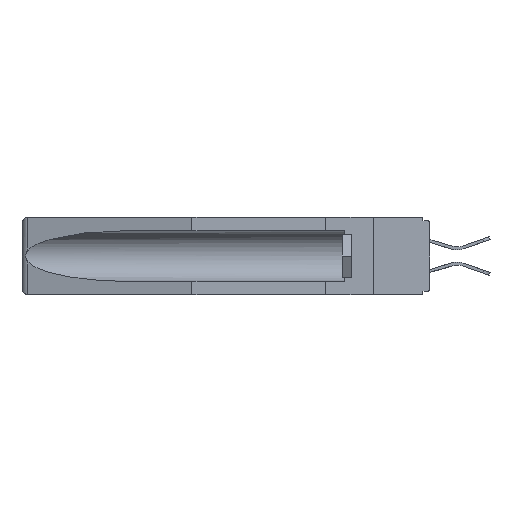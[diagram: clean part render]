
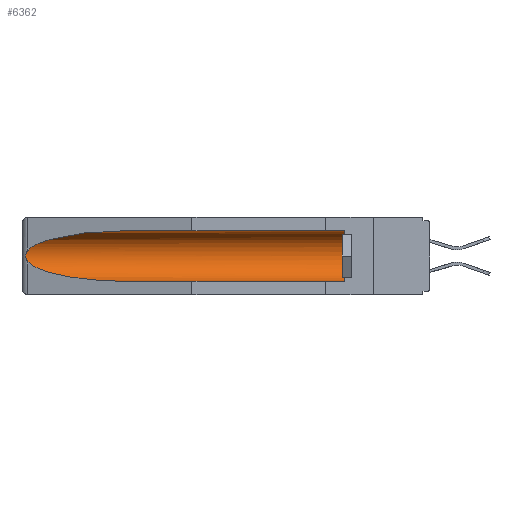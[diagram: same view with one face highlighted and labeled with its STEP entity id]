
A CAD part, left-side view. The second image highlights one B-rep face of the part: STEP entity #6362.
In plain terms, the highlighted cylindrical face has radius 2.857 mm (diameter 5.715 mm), a partial arc.
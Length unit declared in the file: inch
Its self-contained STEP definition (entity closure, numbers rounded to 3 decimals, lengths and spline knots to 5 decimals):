
#786 =( BOUNDED_CURVE ( )  B_SPLINE_CURVE ( 3, ( #9335, #29809, #32373, #17058 ),
 .UNSPECIFIED., .F., .F. ) 
 B_SPLINE_CURVE_WITH_KNOTS ( ( 4, 4 ),
 ( 0.1948, 1.5708 ),
 .UNSPECIFIED. ) 
 CURVE ( )  GEOMETRIC_REPRESENTATION_ITEM ( )  RATIONAL_B_SPLINE_CURVE ( ( 1., 0.848, 0.848, 1. ) ) 
 REPRESENTATION_ITEM ( '' )  );
#1074 = EDGE_CURVE ( 'NONE', #22549, #25839, #786, .T. ) ;
#1960 = DIRECTION ( 'NONE',  ( 0., 1., 0. ) ) ;
#3177 = ORIENTED_EDGE ( 'NONE', *, *, #28253, .F. ) ;
#3243 = AXIS2_PLACEMENT_3D ( 'NONE', #26136, #16090, #18983 ) ;
#4398 = ORIENTED_EDGE ( 'NONE', *, *, #6813, .T. ) ;
#4669 =( BOUNDED_CURVE ( )  B_SPLINE_CURVE ( 3, ( #23177, #28221, #23061, #18161 ),
 .UNSPECIFIED., .F., .F. ) 
 B_SPLINE_CURVE_WITH_KNOTS ( ( 4, 4 ),
 ( 4.71239, 6.08839 ),
 .UNSPECIFIED. ) 
 CURVE ( )  GEOMETRIC_REPRESENTATION_ITEM ( )  RATIONAL_B_SPLINE_CURVE ( ( 1., 0.848, 0.848, 1. ) ) 
 REPRESENTATION_ITEM ( '' )  );
#6097 = CARTESIAN_POINT ( 'NONE',  ( 0.2673, 1.5327, -0.16383 ) ) ;
#6362 = ADVANCED_FACE ( 'NONE', ( #22747 ), #14728, .F. ) ;
#6813 = EDGE_CURVE ( 'NONE', #18980, #8653, #4669, .T. ) ;
#8653 = VERTEX_POINT ( 'NONE', #18486 ) ;
#8875 = CARTESIAN_POINT ( 'NONE',  ( 0.26537, 1.52718, -0.19328 ) ) ;
#9270 = DIRECTION ( 'NONE',  ( 0., 1., 0. ) ) ;
#9335 = CARTESIAN_POINT ( 'NONE',  ( 0.26537, 1.52718, -0.19328 ) ) ;
#9985 = CARTESIAN_POINT ( 'NONE',  ( 0.155, 0.126, -0.284 ) ) ;
#10874 = VECTOR ( 'NONE', #18351, 39.37008 ) ;
#10895 = CARTESIAN_POINT ( 'NONE',  ( 0.155, 1.07973, -0.059 ) ) ;
#11290 = ORIENTED_EDGE ( 'NONE', *, *, #31826, .T. ) ;
#11329 = CARTESIAN_POINT ( 'NONE',  ( 0.26655, 1.53094, -0.18657 ) ) ;
#11536 = CARTESIAN_POINT ( 'NONE',  ( 0.2673, 1.53269, -0.17917 ) ) ;
#12508 = VERTEX_POINT ( 'NONE', #16793 ) ;
#14493 = B_SPLINE_CURVE_WITH_KNOTS ( 'NONE', 3,
 ( #18865, #26876, #31922, #6097, #19180, #16621, #11536, #11329, #26559, #8875 ),
 .UNSPECIFIED., .F., .F.,
 ( 4, 2, 2, 2, 4 ),
 ( 0., 0.00029, 0.00058, 0.00087, 0.00117 ),
 .UNSPECIFIED. ) ;
#14728 = CYLINDRICAL_SURFACE ( 'NONE', #17999, 0.1125 ) ;
#15441 = CARTESIAN_POINT ( 'NONE',  ( 0.155, -0.30754, -0.284 ) ) ;
#15963 = EDGE_LOOP ( 'NONE', ( #4398, #11290, #25491, #3177, #27975, #26094 ) ) ;
#16090 = DIRECTION ( 'NONE',  ( 0., -1., 0. ) ) ;
#16621 = CARTESIAN_POINT ( 'NONE',  ( 0.2675, 1.53308, -0.17534 ) ) ;
#16793 = CARTESIAN_POINT ( 'NONE',  ( 0.155, 0.126, -0.059 ) ) ;
#16887 = EDGE_CURVE ( 'NONE', #31960, #12508, #23638, .T. ) ;
#17058 = CARTESIAN_POINT ( 'NONE',  ( 0.155, 1.07973, -0.284 ) ) ;
#17071 = VECTOR ( 'NONE', #1960, 39.37008 ) ;
#17648 = CARTESIAN_POINT ( 'NONE',  ( 0.155, -0.30754, -0.059 ) ) ;
#17657 = CARTESIAN_POINT ( 'NONE',  ( 0.26537, 1.52718, -0.19328 ) ) ;
#17698 = LINE ( 'NONE', #15441, #10874 ) ;
#17999 = AXIS2_PLACEMENT_3D ( 'NONE', #24587, #9270, #32089 ) ;
#18161 = CARTESIAN_POINT ( 'NONE',  ( 0.26537, 1.52718, -0.14972 ) ) ;
#18351 = DIRECTION ( 'NONE',  ( 0., 1., 0. ) ) ;
#18486 = CARTESIAN_POINT ( 'NONE',  ( 0.26537, 1.52718, -0.14972 ) ) ;
#18865 = CARTESIAN_POINT ( 'NONE',  ( 0.26537, 1.52718, -0.14972 ) ) ;
#18980 = VERTEX_POINT ( 'NONE', #10895 ) ;
#18983 = DIRECTION ( 'NONE',  ( 0., 0., 1. ) ) ;
#19180 = CARTESIAN_POINT ( 'NONE',  ( 0.2675, 1.53308, -0.16763 ) ) ;
#22271 = LINE ( 'NONE', #17648, #17071 ) ;
#22549 = VERTEX_POINT ( 'NONE', #17657 ) ;
#22747 = FACE_OUTER_BOUND ( 'NONE', #15963, .T. ) ;
#23061 = CARTESIAN_POINT ( 'NONE',  ( 0.25451, 1.48313, -0.09465 ) ) ;
#23177 = CARTESIAN_POINT ( 'NONE',  ( 0.155, 1.07973, -0.059 ) ) ;
#23181 = CARTESIAN_POINT ( 'NONE',  ( 0.155, 1.07973, -0.284 ) ) ;
#23638 = CIRCLE ( 'NONE', #3243, 0.1125 ) ;
#24587 = CARTESIAN_POINT ( 'NONE',  ( 0.155, -0.30754, -0.1715 ) ) ;
#25491 = ORIENTED_EDGE ( 'NONE', *, *, #1074, .T. ) ;
#25545 = EDGE_CURVE ( 'NONE', #12508, #18980, #22271, .T. ) ;
#25839 = VERTEX_POINT ( 'NONE', #23181 ) ;
#26094 = ORIENTED_EDGE ( 'NONE', *, *, #25545, .T. ) ;
#26136 = CARTESIAN_POINT ( 'NONE',  ( 0.155, 0.126, -0.1715 ) ) ;
#26559 = CARTESIAN_POINT ( 'NONE',  ( 0.26597, 1.5296, -0.19026 ) ) ;
#26876 = CARTESIAN_POINT ( 'NONE',  ( 0.26597, 1.52961, -0.15275 ) ) ;
#27975 = ORIENTED_EDGE ( 'NONE', *, *, #16887, .T. ) ;
#28221 = CARTESIAN_POINT ( 'NONE',  ( 0.21114, 1.30732, -0.059 ) ) ;
#28253 = EDGE_CURVE ( 'NONE', #31960, #25839, #17698, .T. ) ;
#29809 = CARTESIAN_POINT ( 'NONE',  ( 0.25451, 1.48313, -0.24835 ) ) ;
#31826 = EDGE_CURVE ( 'NONE', #8653, #22549, #14493, .T. ) ;
#31922 = CARTESIAN_POINT ( 'NONE',  ( 0.26654, 1.53092, -0.15636 ) ) ;
#31960 = VERTEX_POINT ( 'NONE', #9985 ) ;
#32089 = DIRECTION ( 'NONE',  ( 0., 0., 1. ) ) ;
#32373 = CARTESIAN_POINT ( 'NONE',  ( 0.21114, 1.30732, -0.284 ) ) ;
